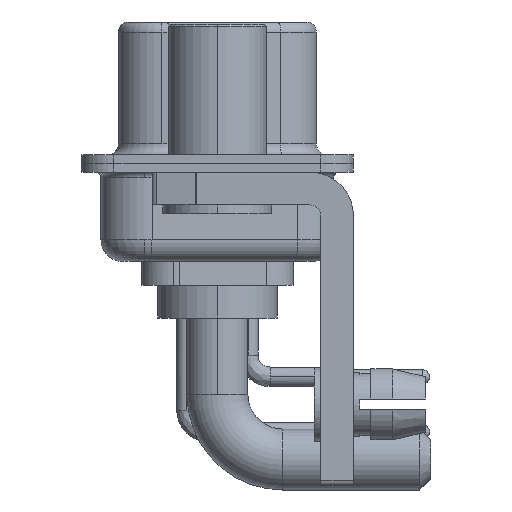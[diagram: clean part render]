
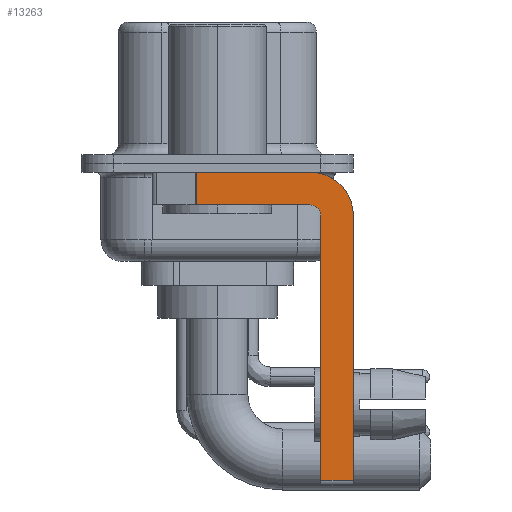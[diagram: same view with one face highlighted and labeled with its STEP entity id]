
A CAD part, left-side view. The second image highlights one B-rep face of the part: STEP entity #13263.
In plain terms, the highlighted planar face has unit normal (-1, 0, 0).
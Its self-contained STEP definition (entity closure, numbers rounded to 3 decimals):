
#266 = DIRECTION ( 'NONE',  ( 1., 0., 0. ) ) ;
#862 = DIRECTION ( 'NONE',  ( -1., 0., 0. ) ) ;
#1032 = LINE ( 'NONE', #9812, #27248 ) ;
#1187 = LINE ( 'NONE', #27762, #12009 ) ;
#1317 = AXIS2_PLACEMENT_3D ( 'NONE', #6707, #266, #27140 ) ;
#2355 = VECTOR ( 'NONE', #4139, 1000. ) ;
#2611 = EDGE_CURVE ( 'NONE', #11711, #2822, #1187, .T. ) ;
#2822 = VERTEX_POINT ( 'NONE', #19564 ) ;
#3226 = DIRECTION ( 'NONE',  ( 0., 1., 0. ) ) ;
#3482 = CARTESIAN_POINT ( 'NONE',  ( -2.9, -4.25, -2.4 ) ) ;
#3612 = DIRECTION ( 'NONE',  ( 0., 0., -1. ) ) ;
#3922 = CIRCLE ( 'NONE', #18834, 0.5 ) ;
#4139 = DIRECTION ( 'NONE',  ( 0., 0., -1. ) ) ;
#4210 = EDGE_CURVE ( 'NONE', #22853, #27127, #26440, .T. ) ;
#4396 = EDGE_LOOP ( 'NONE', ( #10339, #9086, #24720, #16875, #6950, #15017, #25510, #8648 ) ) ;
#4822 = VECTOR ( 'NONE', #11797, 1000. ) ;
#4969 = CARTESIAN_POINT ( 'NONE',  ( -2.9, -4.75, -2.4 ) ) ;
#5463 = EDGE_CURVE ( 'NONE', #19395, #22853, #16706, .T. ) ;
#6707 = CARTESIAN_POINT ( 'NONE',  ( -2.9, -4.25, -2.4 ) ) ;
#6950 = ORIENTED_EDGE ( 'NONE', *, *, #12747, .F. ) ;
#8225 = VECTOR ( 'NONE', #18705, 1000. ) ;
#8232 = LINE ( 'NONE', #17104, #4822 ) ;
#8628 = DIRECTION ( 'NONE',  ( 0., 0., -1. ) ) ;
#8648 = ORIENTED_EDGE ( 'NONE', *, *, #5463, .F. ) ;
#9086 = ORIENTED_EDGE ( 'NONE', *, *, #23568, .T. ) ;
#9812 = CARTESIAN_POINT ( 'NONE',  ( -2.9, -4.75, -14.8 ) ) ;
#10339 = ORIENTED_EDGE ( 'NONE', *, *, #17346, .F. ) ;
#10703 = CARTESIAN_POINT ( 'NONE',  ( -2.9, -4.25, -0.4 ) ) ;
#10789 = CARTESIAN_POINT ( 'NONE',  ( -2.9, 0.978, -0.4 ) ) ;
#11028 = CARTESIAN_POINT ( 'NONE',  ( -2.9, -4.25, -2.4 ) ) ;
#11711 = VERTEX_POINT ( 'NONE', #12631 ) ;
#11797 = DIRECTION ( 'NONE',  ( 0., -1., 0. ) ) ;
#11852 = EDGE_CURVE ( 'NONE', #13097, #27127, #8232, .T. ) ;
#12009 = VECTOR ( 'NONE', #3226, 1000. ) ;
#12631 = CARTESIAN_POINT ( 'NONE',  ( -2.9, -4.25, -1.9 ) ) ;
#12747 = EDGE_CURVE ( 'NONE', #13097, #24065, #1032, .T. ) ;
#13097 = VERTEX_POINT ( 'NONE', #16165 ) ;
#13263 = ADVANCED_FACE ( 'NONE', ( #28011 ), #22252, .F. ) ;
#14190 = EDGE_CURVE ( 'NONE', #24065, #11711, #3922, .T. ) ;
#14412 = VERTEX_POINT ( 'NONE', #10789 ) ;
#15017 = ORIENTED_EDGE ( 'NONE', *, *, #11852, .T. ) ;
#15184 = CARTESIAN_POINT ( 'NONE',  ( -2.9, -6.25, -2.4 ) ) ;
#15787 = LINE ( 'NONE', #17545, #2355 ) ;
#16165 = CARTESIAN_POINT ( 'NONE',  ( -2.9, -4.75, -14.55 ) ) ;
#16654 = CARTESIAN_POINT ( 'NONE',  ( -2.9, 3., -0.4 ) ) ;
#16706 = CIRCLE ( 'NONE', #1317, 2. ) ;
#16875 = ORIENTED_EDGE ( 'NONE', *, *, #14190, .F. ) ;
#17029 = CARTESIAN_POINT ( 'NONE',  ( -2.9, -6.25, -2.4 ) ) ;
#17104 = CARTESIAN_POINT ( 'NONE',  ( -2.9, -4.25, -14.55 ) ) ;
#17346 = EDGE_CURVE ( 'NONE', #14412, #19395, #23546, .T. ) ;
#17545 = CARTESIAN_POINT ( 'NONE',  ( -2.9, 0.978, -1.9 ) ) ;
#18705 = DIRECTION ( 'NONE',  ( 0., -1., 0. ) ) ;
#18834 = AXIS2_PLACEMENT_3D ( 'NONE', #3482, #862, #25250 ) ;
#19395 = VERTEX_POINT ( 'NONE', #10703 ) ;
#19564 = CARTESIAN_POINT ( 'NONE',  ( -2.9, 0.978, -1.9 ) ) ;
#21195 = AXIS2_PLACEMENT_3D ( 'NONE', #11028, #21425, #3612 ) ;
#21425 = DIRECTION ( 'NONE',  ( 1., 0., 0. ) ) ;
#22252 = PLANE ( 'NONE',  #21195 ) ;
#22780 = CARTESIAN_POINT ( 'NONE',  ( -2.9, -6.25, -14.55 ) ) ;
#22853 = VERTEX_POINT ( 'NONE', #17029 ) ;
#23546 = LINE ( 'NONE', #16654, #8225 ) ;
#23568 = EDGE_CURVE ( 'NONE', #14412, #2822, #15787, .T. ) ;
#24065 = VERTEX_POINT ( 'NONE', #4969 ) ;
#24720 = ORIENTED_EDGE ( 'NONE', *, *, #2611, .F. ) ;
#25250 = DIRECTION ( 'NONE',  ( 0., 0., 1. ) ) ;
#25510 = ORIENTED_EDGE ( 'NONE', *, *, #4210, .F. ) ;
#26440 = LINE ( 'NONE', #15184, #26968 ) ;
#26968 = VECTOR ( 'NONE', #8628, 1000. ) ;
#27127 = VERTEX_POINT ( 'NONE', #22780 ) ;
#27140 = DIRECTION ( 'NONE',  ( 0., 0., -1. ) ) ;
#27248 = VECTOR ( 'NONE', #27615, 1000. ) ;
#27615 = DIRECTION ( 'NONE',  ( 0., 0., 1. ) ) ;
#27762 = CARTESIAN_POINT ( 'NONE',  ( -2.9, -4.25, -1.9 ) ) ;
#28011 = FACE_OUTER_BOUND ( 'NONE', #4396, .T. ) ;
